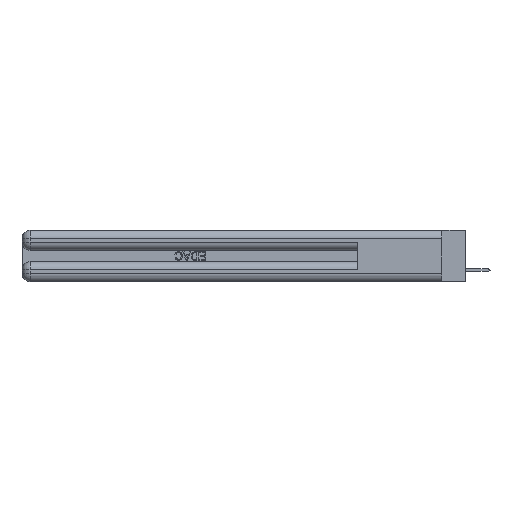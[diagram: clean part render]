
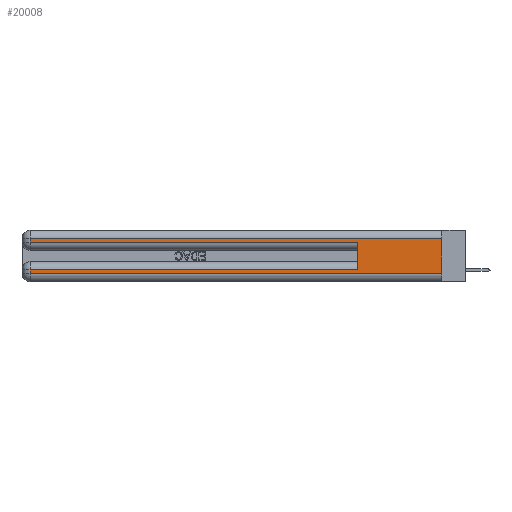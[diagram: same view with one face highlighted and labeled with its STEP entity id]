
A CAD part, left-side view. The second image highlights one B-rep face of the part: STEP entity #20008.
In plain terms, the highlighted planar face has unit normal (-1, 0, 0).
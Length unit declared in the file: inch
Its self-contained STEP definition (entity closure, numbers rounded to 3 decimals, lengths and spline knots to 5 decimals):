
#551 = DIRECTION ( 'NONE',  ( 0., 0., 1. ) ) ;
#797 = CARTESIAN_POINT ( 'NONE',  ( 0., 2.94, 0.285 ) ) ;
#2215 = VECTOR ( 'NONE', #34925, 39.37008 ) ;
#2342 = VERTEX_POINT ( 'NONE', #17457 ) ;
#3208 = CARTESIAN_POINT ( 'NONE',  ( 0., 0., 0.31 ) ) ;
#3570 = CARTESIAN_POINT ( 'NONE',  ( 0., 0., 0.31 ) ) ;
#5017 = LINE ( 'NONE', #36068, #15281 ) ;
#5361 = LINE ( 'NONE', #17571, #9589 ) ;
#5427 = DIRECTION ( 'NONE',  ( 0., 1., 0. ) ) ;
#5645 = LINE ( 'NONE', #3570, #11737 ) ;
#5966 = ORIENTED_EDGE ( 'NONE', *, *, #19483, .T. ) ;
#6921 = DIRECTION ( 'NONE',  ( 0., 1., 0. ) ) ;
#7573 = VERTEX_POINT ( 'NONE', #3208 ) ;
#9059 = EDGE_CURVE ( 'NONE', #7573, #2342, #12503, .T. ) ;
#9065 = PLANE ( 'NONE',  #16624 ) ;
#9589 = VECTOR ( 'NONE', #5427, 39.37008 ) ;
#11592 = CARTESIAN_POINT ( 'NONE',  ( 0., 2.94, 0.37 ) ) ;
#11737 = VECTOR ( 'NONE', #6921, 39.37008 ) ;
#12503 = LINE ( 'NONE', #46898, #2215 ) ;
#15281 = VECTOR ( 'NONE', #22589, 39.37008 ) ;
#15794 = ORIENTED_EDGE ( 'NONE', *, *, #49819, .F. ) ;
#16514 = VERTEX_POINT ( 'NONE', #17103 ) ;
#16624 = AXIS2_PLACEMENT_3D ( 'NONE', #16790, #40416, #17467 ) ;
#16790 = CARTESIAN_POINT ( 'NONE',  ( 0., 0., 0.37 ) ) ;
#17103 = CARTESIAN_POINT ( 'NONE',  ( 0., 2.94, 0.31 ) ) ;
#17457 = CARTESIAN_POINT ( 'NONE',  ( 0., 0., 0.06 ) ) ;
#17467 = DIRECTION ( 'NONE',  ( 0., 0., -1. ) ) ;
#17571 = CARTESIAN_POINT ( 'NONE',  ( 0., 0., 0.085 ) ) ;
#17619 = ORIENTED_EDGE ( 'NONE', *, *, #9059, .F. ) ;
#18792 = CARTESIAN_POINT ( 'NONE',  ( 0., 2.94, 0.06 ) ) ;
#19242 = VERTEX_POINT ( 'NONE', #39035 ) ;
#19483 = EDGE_CURVE ( 'NONE', #23554, #2342, #5017, .T. ) ;
#20008 = ADVANCED_FACE ( 'NONE', ( #32758 ), #9065, .F. ) ;
#20229 = VERTEX_POINT ( 'NONE', #21303 ) ;
#20465 = VERTEX_POINT ( 'NONE', #797 ) ;
#21303 = CARTESIAN_POINT ( 'NONE',  ( 0., 0.6, 0.285 ) ) ;
#21743 = LINE ( 'NONE', #11592, #23584 ) ;
#22520 = CARTESIAN_POINT ( 'NONE',  ( 0., 2.94, 0.37 ) ) ;
#22589 = DIRECTION ( 'NONE',  ( 0., -1., 0. ) ) ;
#22648 = VECTOR ( 'NONE', #47670, 39.37008 ) ;
#23224 = LINE ( 'NONE', #23857, #45579 ) ;
#23554 = VERTEX_POINT ( 'NONE', #18792 ) ;
#23584 = VECTOR ( 'NONE', #37911, 39.37008 ) ;
#23857 = CARTESIAN_POINT ( 'NONE',  ( 0., 0.6, 0.145 ) ) ;
#25465 = EDGE_CURVE ( 'NONE', #7573, #16514, #5645, .T. ) ;
#25823 = VERTEX_POINT ( 'NONE', #32162 ) ;
#26138 = ORIENTED_EDGE ( 'NONE', *, *, #41431, .T. ) ;
#28031 = EDGE_CURVE ( 'NONE', #19242, #25823, #5361, .T. ) ;
#32162 = CARTESIAN_POINT ( 'NONE',  ( 0., 2.94, 0.085 ) ) ;
#32743 = EDGE_CURVE ( 'NONE', #25823, #23554, #21743, .T. ) ;
#32758 = FACE_OUTER_BOUND ( 'NONE', #33938, .T. ) ;
#33938 = EDGE_LOOP ( 'NONE', ( #17619, #48686, #45021, #26138, #15794, #45999, #46127, #5966 ) ) ;
#34925 = DIRECTION ( 'NONE',  ( 0., 0., -1. ) ) ;
#35852 = LINE ( 'NONE', #47163, #22648 ) ;
#36068 = CARTESIAN_POINT ( 'NONE',  ( 0., 0., 0.06 ) ) ;
#37911 = DIRECTION ( 'NONE',  ( 0., 0., -1. ) ) ;
#39035 = CARTESIAN_POINT ( 'NONE',  ( 0., 0.6, 0.085 ) ) ;
#39557 = VECTOR ( 'NONE', #48239, 39.37008 ) ;
#40416 = DIRECTION ( 'NONE',  ( 1., 0., 0. ) ) ;
#41431 = EDGE_CURVE ( 'NONE', #20465, #20229, #35852, .T. ) ;
#44414 = LINE ( 'NONE', #22520, #39557 ) ;
#45021 = ORIENTED_EDGE ( 'NONE', *, *, #47242, .T. ) ;
#45579 = VECTOR ( 'NONE', #551, 39.37008 ) ;
#45999 = ORIENTED_EDGE ( 'NONE', *, *, #28031, .T. ) ;
#46127 = ORIENTED_EDGE ( 'NONE', *, *, #32743, .T. ) ;
#46898 = CARTESIAN_POINT ( 'NONE',  ( 0., 0., 0.37 ) ) ;
#47163 = CARTESIAN_POINT ( 'NONE',  ( 0., 0., 0.285 ) ) ;
#47242 = EDGE_CURVE ( 'NONE', #16514, #20465, #44414, .T. ) ;
#47670 = DIRECTION ( 'NONE',  ( 0., -1., 0. ) ) ;
#48239 = DIRECTION ( 'NONE',  ( 0., 0., -1. ) ) ;
#48686 = ORIENTED_EDGE ( 'NONE', *, *, #25465, .T. ) ;
#49819 = EDGE_CURVE ( 'NONE', #19242, #20229, #23224, .T. ) ;
